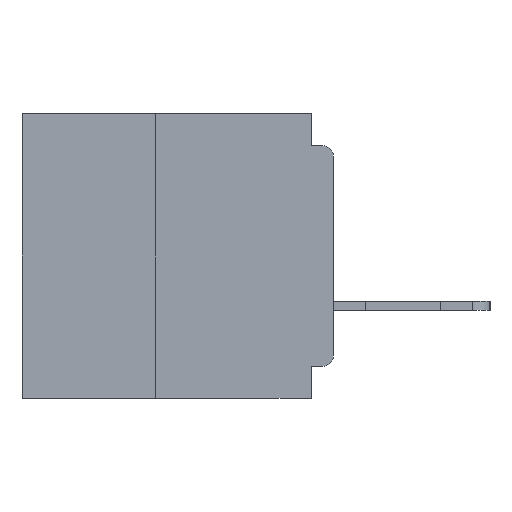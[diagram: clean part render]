
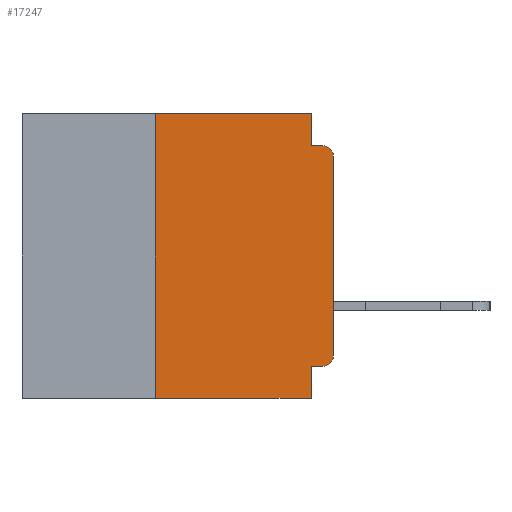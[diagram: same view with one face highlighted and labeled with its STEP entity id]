
A CAD part, left-side view. The second image highlights one B-rep face of the part: STEP entity #17247.
In plain terms, the highlighted planar face has unit normal (-1, 0, 0).
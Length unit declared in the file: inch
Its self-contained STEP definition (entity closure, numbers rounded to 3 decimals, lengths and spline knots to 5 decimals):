
#402 = EDGE_CURVE ( 'NONE', #17259, #33085, #31781, .T. ) ;
#1521 = EDGE_CURVE ( 'NONE', #15368, #21739, #15048, .T. ) ;
#1571 = DIRECTION ( 'NONE',  ( -1., 0., 0. ) ) ;
#2577 = EDGE_CURVE ( 'NONE', #15524, #10967, #14453, .T. ) ;
#2939 = LINE ( 'NONE', #5099, #18219 ) ;
#3141 = VECTOR ( 'NONE', #24428, 39.37008 ) ;
#3610 = CARTESIAN_POINT ( 'NONE',  ( 0., 0.25, 0. ) ) ;
#3653 = CARTESIAN_POINT ( 'NONE',  ( 0., 0.015, -0.34 ) ) ;
#3962 = CARTESIAN_POINT ( 'NONE',  ( 0., 0., -0.34 ) ) ;
#4874 = DIRECTION ( 'NONE',  ( 0., 0., 1. ) ) ;
#5099 = CARTESIAN_POINT ( 'NONE',  ( 0., 0.437, -0.4 ) ) ;
#5102 = EDGE_CURVE ( 'NONE', #33085, #15524, #32074, .T. ) ;
#5153 = DIRECTION ( 'NONE',  ( 0., 0., -1. ) ) ;
#5800 = VECTOR ( 'NONE', #8203, 39.37008 ) ;
#6908 = ORIENTED_EDGE ( 'NONE', *, *, #2577, .F. ) ;
#6950 = DIRECTION ( 'NONE',  ( 0., 0., -1. ) ) ;
#7143 = VECTOR ( 'NONE', #40413, 39.37008 ) ;
#8147 = CARTESIAN_POINT ( 'NONE',  ( 0., 0.031, -0.045 ) ) ;
#8203 = DIRECTION ( 'NONE',  ( 0., 0., -1. ) ) ;
#10967 = VERTEX_POINT ( 'NONE', #8147 ) ;
#11565 = AXIS2_PLACEMENT_3D ( 'NONE', #18097, #24659, #5153 ) ;
#12295 = AXIS2_PLACEMENT_3D ( 'NONE', #3653, #26442, #6950 ) ;
#12879 = ORIENTED_EDGE ( 'NONE', *, *, #36205, .T. ) ;
#13899 = DIRECTION ( 'NONE',  ( 0., -1., 0. ) ) ;
#14087 = ORIENTED_EDGE ( 'NONE', *, *, #5102, .F. ) ;
#14453 = LINE ( 'NONE', #21155, #5800 ) ;
#14633 = EDGE_LOOP ( 'NONE', ( #18775, #17523, #34835, #6908, #14087, #14698, #12879, #34286, #29916, #19219 ) ) ;
#14698 = ORIENTED_EDGE ( 'NONE', *, *, #402, .F. ) ;
#15048 = LINE ( 'NONE', #41590, #40076 ) ;
#15368 = VERTEX_POINT ( 'NONE', #38798 ) ;
#15524 = VERTEX_POINT ( 'NONE', #36386 ) ;
#16642 = DIRECTION ( 'NONE',  ( 0., 1., 0. ) ) ;
#17247 = ADVANCED_FACE ( 'NONE', ( #38151 ), #34381, .F. ) ;
#17259 = VERTEX_POINT ( 'NONE', #28087 ) ;
#17523 = ORIENTED_EDGE ( 'NONE', *, *, #35128, .T. ) ;
#17590 = CARTESIAN_POINT ( 'NONE',  ( 0., 0.437, 0. ) ) ;
#17879 = CARTESIAN_POINT ( 'NONE',  ( 0., 0.015, -0.045 ) ) ;
#18097 = CARTESIAN_POINT ( 'NONE',  ( 0., 0.437, 0. ) ) ;
#18219 = VECTOR ( 'NONE', #24602, 39.37008 ) ;
#18665 = CIRCLE ( 'NONE', #12295, 0.015 ) ;
#18775 = ORIENTED_EDGE ( 'NONE', *, *, #36506, .T. ) ;
#19219 = ORIENTED_EDGE ( 'NONE', *, *, #30721, .T. ) ;
#19625 = DIRECTION ( 'NONE',  ( 0., 0., 1. ) ) ;
#19890 = CIRCLE ( 'NONE', #39447, 0.015 ) ;
#20495 = LINE ( 'NONE', #37431, #3141 ) ;
#21072 = CARTESIAN_POINT ( 'NONE',  ( 0., 0.015, -0.06 ) ) ;
#21155 = CARTESIAN_POINT ( 'NONE',  ( 0., 0.031, 0. ) ) ;
#21739 = VERTEX_POINT ( 'NONE', #26898 ) ;
#23366 = EDGE_CURVE ( 'NONE', #10967, #33984, #24422, .T. ) ;
#23700 = CARTESIAN_POINT ( 'NONE',  ( 0., 0., -0.045 ) ) ;
#24140 = VECTOR ( 'NONE', #4874, 39.37008 ) ;
#24348 = DIRECTION ( 'NONE',  ( 0., 0., -1. ) ) ;
#24422 = LINE ( 'NONE', #23700, #39766 ) ;
#24428 = DIRECTION ( 'NONE',  ( 0., 0., -1. ) ) ;
#24602 = DIRECTION ( 'NONE',  ( 0., -1., 0. ) ) ;
#24659 = DIRECTION ( 'NONE',  ( 1., 0., 0. ) ) ;
#26442 = DIRECTION ( 'NONE',  ( -1., 0., 0. ) ) ;
#26898 = CARTESIAN_POINT ( 'NONE',  ( 0., 0.031, -0.355 ) ) ;
#27378 = CARTESIAN_POINT ( 'NONE',  ( 0., 0.25, -0.4 ) ) ;
#28087 = CARTESIAN_POINT ( 'NONE',  ( 0., 0.25, -0.4 ) ) ;
#29438 = CARTESIAN_POINT ( 'NONE',  ( 0., 0., 0. ) ) ;
#29916 = ORIENTED_EDGE ( 'NONE', *, *, #1521, .F. ) ;
#30601 = VERTEX_POINT ( 'NONE', #35325 ) ;
#30721 = EDGE_CURVE ( 'NONE', #15368, #40534, #18665, .T. ) ;
#31781 = LINE ( 'NONE', #27378, #24140 ) ;
#31802 = VERTEX_POINT ( 'NONE', #35503 ) ;
#32074 = LINE ( 'NONE', #17590, #7143 ) ;
#33085 = VERTEX_POINT ( 'NONE', #3610 ) ;
#33984 = VERTEX_POINT ( 'NONE', #17879 ) ;
#33987 = EDGE_CURVE ( 'NONE', #21739, #31802, #20495, .T. ) ;
#34286 = ORIENTED_EDGE ( 'NONE', *, *, #33987, .F. ) ;
#34381 = PLANE ( 'NONE',  #11565 ) ;
#34835 = ORIENTED_EDGE ( 'NONE', *, *, #23366, .F. ) ;
#35128 = EDGE_CURVE ( 'NONE', #30601, #33984, #19890, .T. ) ;
#35325 = CARTESIAN_POINT ( 'NONE',  ( 0., 0., -0.06 ) ) ;
#35503 = CARTESIAN_POINT ( 'NONE',  ( 0., 0.031, -0.4 ) ) ;
#36205 = EDGE_CURVE ( 'NONE', #17259, #31802, #2939, .T. ) ;
#36386 = CARTESIAN_POINT ( 'NONE',  ( 0., 0.031, 0. ) ) ;
#36506 = EDGE_CURVE ( 'NONE', #40534, #30601, #40669, .T. ) ;
#37431 = CARTESIAN_POINT ( 'NONE',  ( 0., 0.031, -0.4 ) ) ;
#38151 = FACE_OUTER_BOUND ( 'NONE', #14633, .T. ) ;
#38798 = CARTESIAN_POINT ( 'NONE',  ( 0., 0.015, -0.355 ) ) ;
#39447 = AXIS2_PLACEMENT_3D ( 'NONE', #21072, #1571, #24348 ) ;
#39766 = VECTOR ( 'NONE', #13899, 39.37008 ) ;
#40076 = VECTOR ( 'NONE', #16642, 39.37008 ) ;
#40413 = DIRECTION ( 'NONE',  ( 0., -1., 0. ) ) ;
#40534 = VERTEX_POINT ( 'NONE', #3962 ) ;
#40669 = LINE ( 'NONE', #29438, #41203 ) ;
#41203 = VECTOR ( 'NONE', #19625, 39.37008 ) ;
#41590 = CARTESIAN_POINT ( 'NONE',  ( 0., 0., -0.355 ) ) ;
